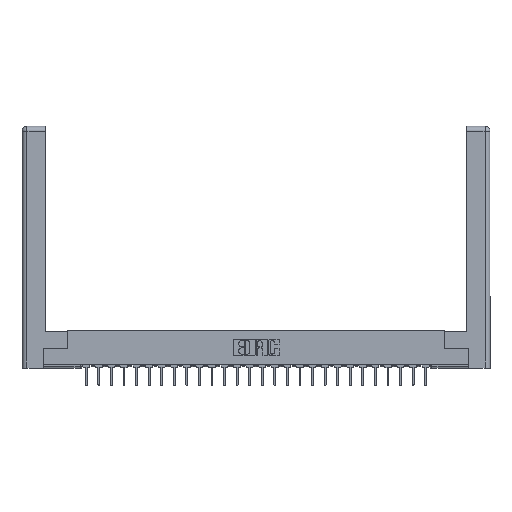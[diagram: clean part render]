
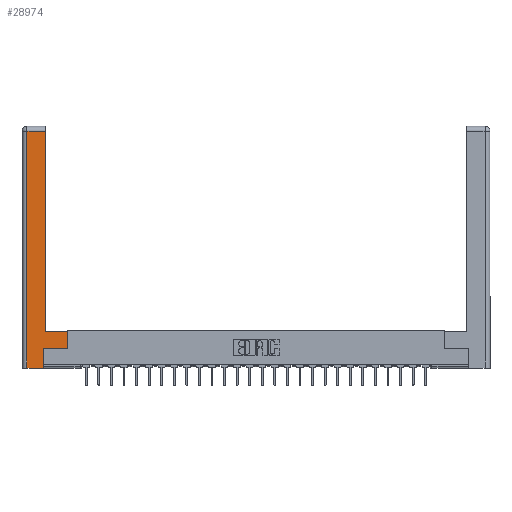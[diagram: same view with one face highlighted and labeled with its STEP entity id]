
A CAD part, top view. The second image highlights one B-rep face of the part: STEP entity #28974.
In plain terms, the highlighted planar face has unit normal (0, 0, 1).
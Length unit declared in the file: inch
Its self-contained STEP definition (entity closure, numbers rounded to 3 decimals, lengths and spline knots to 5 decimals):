
#425 = ORIENTED_EDGE ( 'NONE', *, *, #7896, .T. ) ;
#724 = VECTOR ( 'NONE', #3676, 39.37008 ) ;
#945 = VECTOR ( 'NONE', #11981, 39.37008 ) ;
#1026 = CARTESIAN_POINT ( 'NONE',  ( 0.565, 0.245, 0. ) ) ;
#2620 = CARTESIAN_POINT ( 'NONE',  ( 0.265, 0., 0. ) ) ;
#2997 = CARTESIAN_POINT ( 'NONE',  ( 0.565, 0.245, 0. ) ) ;
#3122 = DIRECTION ( 'NONE',  ( 0., 1., 0. ) ) ;
#3676 = DIRECTION ( 'NONE',  ( -1., 0., 0. ) ) ;
#3782 = EDGE_CURVE ( 'NONE', #4628, #6826, #28504, .T. ) ;
#4164 = VECTOR ( 'NONE', #24770, 39.37008 ) ;
#4518 = CARTESIAN_POINT ( 'NONE',  ( 0.295, 3., 0. ) ) ;
#4628 = VERTEX_POINT ( 'NONE', #6241 ) ;
#4784 = DIRECTION ( 'NONE',  ( 1., 0., 0. ) ) ;
#4944 = VERTEX_POINT ( 'NONE', #5334 ) ;
#5186 = PLANE ( 'NONE',  #14410 ) ;
#5212 = ORIENTED_EDGE ( 'NONE', *, *, #24830, .T. ) ;
#5334 = CARTESIAN_POINT ( 'NONE',  ( 0.565, 0.45, 0. ) ) ;
#5376 = CARTESIAN_POINT ( 'NONE',  ( 0.265, 0.245, 0. ) ) ;
#5610 = VERTEX_POINT ( 'NONE', #21121 ) ;
#5804 = EDGE_LOOP ( 'NONE', ( #7469, #5212, #425, #21220, #27258, #12271, #10447, #15663 ) ) ;
#6241 = CARTESIAN_POINT ( 'NONE',  ( 0.265, 0.245, 0. ) ) ;
#6769 = CARTESIAN_POINT ( 'NONE',  ( 0.0615, 2.94, 0. ) ) ;
#6826 = VERTEX_POINT ( 'NONE', #1026 ) ;
#7065 = CARTESIAN_POINT ( 'NONE',  ( 0.295, 0.45, 0. ) ) ;
#7463 = DIRECTION ( 'NONE',  ( 0., 0., -1. ) ) ;
#7469 = ORIENTED_EDGE ( 'NONE', *, *, #16192, .T. ) ;
#7568 = EDGE_CURVE ( 'NONE', #4944, #19342, #20152, .T. ) ;
#7896 = EDGE_CURVE ( 'NONE', #9913, #24940, #28267, .T. ) ;
#8138 = CARTESIAN_POINT ( 'NONE',  ( 0.0615, 2.94, 0. ) ) ;
#8266 = LINE ( 'NONE', #19227, #20584 ) ;
#9747 = DIRECTION ( 'NONE',  ( -1., 0., 0. ) ) ;
#9873 = EDGE_CURVE ( 'NONE', #24940, #28979, #16986, .T. ) ;
#9913 = VERTEX_POINT ( 'NONE', #6769 ) ;
#10447 = ORIENTED_EDGE ( 'NONE', *, *, #23378, .T. ) ;
#11380 = CARTESIAN_POINT ( 'NONE',  ( 0.0615, 0., 0. ) ) ;
#11981 = DIRECTION ( 'NONE',  ( 0., 1., 0. ) ) ;
#12271 = ORIENTED_EDGE ( 'NONE', *, *, #3782, .T. ) ;
#13148 = EDGE_CURVE ( 'NONE', #28979, #4628, #22838, .T. ) ;
#14015 = LINE ( 'NONE', #4518, #4164 ) ;
#14385 = DIRECTION ( 'NONE',  ( -1., 0., 0. ) ) ;
#14410 = AXIS2_PLACEMENT_3D ( 'NONE', #21009, #7463, #9747 ) ;
#15663 = ORIENTED_EDGE ( 'NONE', *, *, #7568, .T. ) ;
#16192 = EDGE_CURVE ( 'NONE', #19342, #5610, #14015, .T. ) ;
#16986 = LINE ( 'NONE', #27310, #27590 ) ;
#18265 = DIRECTION ( 'NONE',  ( 0., -1., 0. ) ) ;
#19227 = CARTESIAN_POINT ( 'NONE',  ( 0.565, 0.45, 0. ) ) ;
#19342 = VERTEX_POINT ( 'NONE', #7065 ) ;
#20152 = LINE ( 'NONE', #28337, #27562 ) ;
#20356 = CARTESIAN_POINT ( 'NONE',  ( 0.0615, 0., 0. ) ) ;
#20584 = VECTOR ( 'NONE', #3122, 39.37008 ) ;
#21009 = CARTESIAN_POINT ( 'NONE',  ( 0., 0., 0. ) ) ;
#21121 = CARTESIAN_POINT ( 'NONE',  ( 0.295, 2.94, 0. ) ) ;
#21220 = ORIENTED_EDGE ( 'NONE', *, *, #9873, .T. ) ;
#22261 = VECTOR ( 'NONE', #18265, 39.37008 ) ;
#22838 = LINE ( 'NONE', #5376, #945 ) ;
#23378 = EDGE_CURVE ( 'NONE', #6826, #4944, #8266, .T. ) ;
#24740 = LINE ( 'NONE', #8138, #724 ) ;
#24770 = DIRECTION ( 'NONE',  ( 0., 1., 0. ) ) ;
#24830 = EDGE_CURVE ( 'NONE', #5610, #9913, #24740, .T. ) ;
#24940 = VERTEX_POINT ( 'NONE', #20356 ) ;
#25533 = DIRECTION ( 'NONE',  ( 1., 0., 0. ) ) ;
#27044 = VECTOR ( 'NONE', #25533, 39.37008 ) ;
#27258 = ORIENTED_EDGE ( 'NONE', *, *, #13148, .T. ) ;
#27310 = CARTESIAN_POINT ( 'NONE',  ( 0.265, 0., 0. ) ) ;
#27562 = VECTOR ( 'NONE', #14385, 39.37008 ) ;
#27590 = VECTOR ( 'NONE', #4784, 39.37008 ) ;
#28267 = LINE ( 'NONE', #11380, #22261 ) ;
#28337 = CARTESIAN_POINT ( 'NONE',  ( 0.295, 0.45, 0. ) ) ;
#28504 = LINE ( 'NONE', #2997, #27044 ) ;
#28974 = ADVANCED_FACE ( 'NONE', ( #29121 ), #5186, .F. ) ;
#28979 = VERTEX_POINT ( 'NONE', #2620 ) ;
#29121 = FACE_OUTER_BOUND ( 'NONE', #5804, .T. ) ;
